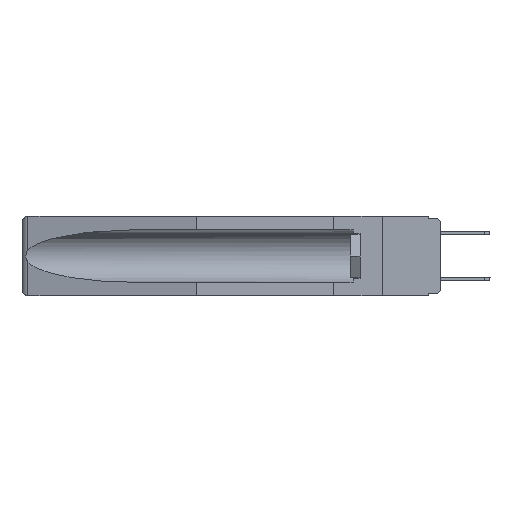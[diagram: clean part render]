
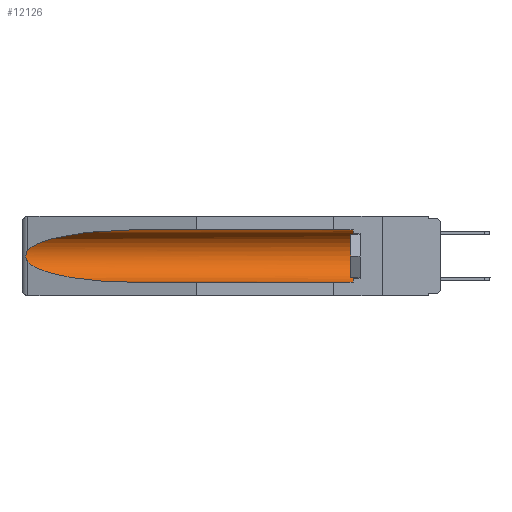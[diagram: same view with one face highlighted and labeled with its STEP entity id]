
A CAD part, left-side view. The second image highlights one B-rep face of the part: STEP entity #12126.
In plain terms, the highlighted cylindrical face has radius 2.857 mm (diameter 5.715 mm), a partial arc.
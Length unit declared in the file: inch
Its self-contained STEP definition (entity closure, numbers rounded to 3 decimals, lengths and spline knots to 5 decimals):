
#92 = CARTESIAN_POINT ( 'NONE',  ( 0.26597, 1.5296, -0.19026 ) ) ;
#160 = CARTESIAN_POINT ( 'NONE',  ( 0.2675, 1.53308, -0.17534 ) ) ;
#314 = CARTESIAN_POINT ( 'NONE',  ( 0.21114, 1.30732, -0.284 ) ) ;
#793 = CARTESIAN_POINT ( 'NONE',  ( 0.26537, 1.52718, -0.14972 ) ) ;
#815 = VERTEX_POINT ( 'NONE', #5006 ) ;
#1790 = CARTESIAN_POINT ( 'NONE',  ( 0.2673, 1.5327, -0.16383 ) ) ;
#1951 = CARTESIAN_POINT ( 'NONE',  ( 0.155, 1.07973, -0.284 ) ) ;
#2643 = CIRCLE ( 'NONE', #19537, 0.1125 ) ;
#2951 = CARTESIAN_POINT ( 'NONE',  ( 0.155, 0.126, -0.1715 ) ) ;
#3215 = CARTESIAN_POINT ( 'NONE',  ( 0.155, -0.30754, -0.1715 ) ) ;
#3278 = LINE ( 'NONE', #11334, #18023 ) ;
#3651 = VERTEX_POINT ( 'NONE', #17450 ) ;
#4057 = VERTEX_POINT ( 'NONE', #12811 ) ;
#5006 = CARTESIAN_POINT ( 'NONE',  ( 0.155, 0.126, -0.059 ) ) ;
#6608 = DIRECTION ( 'NONE',  ( 0., 1., 0. ) ) ;
#6919 = CARTESIAN_POINT ( 'NONE',  ( 0.2675, 1.53308, -0.16763 ) ) ;
#7635 = ORIENTED_EDGE ( 'NONE', *, *, #14720, .T. ) ;
#7788 = ORIENTED_EDGE ( 'NONE', *, *, #12703, .T. ) ;
#8964 = VECTOR ( 'NONE', #14452, 39.37008 ) ;
#8968 =( BOUNDED_CURVE ( )  B_SPLINE_CURVE ( 3, ( #12508, #19167, #314, #1951 ),
 .UNSPECIFIED., .F., .F. ) 
 B_SPLINE_CURVE_WITH_KNOTS ( ( 4, 4 ),
 ( 0.1948, 1.5708 ),
 .UNSPECIFIED. ) 
 CURVE ( )  GEOMETRIC_REPRESENTATION_ITEM ( )  RATIONAL_B_SPLINE_CURVE ( ( 1., 0.848, 0.848, 1. ) ) 
 REPRESENTATION_ITEM ( '' )  );
#9382 = CARTESIAN_POINT ( 'NONE',  ( 0.21114, 1.30732, -0.059 ) ) ;
#10629 = CARTESIAN_POINT ( 'NONE',  ( 0.26537, 1.52718, -0.14972 ) ) ;
#10839 = VERTEX_POINT ( 'NONE', #17985 ) ;
#11134 = CARTESIAN_POINT ( 'NONE',  ( 0.25451, 1.48313, -0.09465 ) ) ;
#11334 = CARTESIAN_POINT ( 'NONE',  ( 0.155, -0.30754, -0.284 ) ) ;
#11445 = ORIENTED_EDGE ( 'NONE', *, *, #18980, .F. ) ;
#12054 = CARTESIAN_POINT ( 'NONE',  ( 0.26597, 1.52961, -0.15275 ) ) ;
#12126 = ADVANCED_FACE ( 'NONE', ( #15658 ), #19638, .F. ) ;
#12508 = CARTESIAN_POINT ( 'NONE',  ( 0.26537, 1.52718, -0.19328 ) ) ;
#12614 = CARTESIAN_POINT ( 'NONE',  ( 0.155, -0.30754, -0.059 ) ) ;
#12703 = EDGE_CURVE ( 'NONE', #815, #10839, #21797, .T. ) ;
#12811 = CARTESIAN_POINT ( 'NONE',  ( 0.26537, 1.52718, -0.19328 ) ) ;
#12832 = CARTESIAN_POINT ( 'NONE',  ( 0.155, 0.126, -0.284 ) ) ;
#12970 =( BOUNDED_CURVE ( )  B_SPLINE_CURVE ( 3, ( #19812, #9382, #11134, #793 ),
 .UNSPECIFIED., .F., .F. ) 
 B_SPLINE_CURVE_WITH_KNOTS ( ( 4, 4 ),
 ( 4.71239, 6.08839 ),
 .UNSPECIFIED. ) 
 CURVE ( )  GEOMETRIC_REPRESENTATION_ITEM ( )  RATIONAL_B_SPLINE_CURVE ( ( 1., 0.848, 0.848, 1. ) ) 
 REPRESENTATION_ITEM ( '' )  );
#13004 = ORIENTED_EDGE ( 'NONE', *, *, #19296, .T. ) ;
#13380 = DIRECTION ( 'NONE',  ( 0., 0., 1. ) ) ;
#13410 = DIRECTION ( 'NONE',  ( 0., -1., 0. ) ) ;
#13753 = CARTESIAN_POINT ( 'NONE',  ( 0.26654, 1.53092, -0.15636 ) ) ;
#13921 = B_SPLINE_CURVE_WITH_KNOTS ( 'NONE', 3,
 ( #10629, #12054, #13753, #1790, #6919, #160, #17448, #18860, #92, #15694 ),
 .UNSPECIFIED., .F., .F.,
 ( 4, 2, 2, 2, 4 ),
 ( 0., 0.00029, 0.00058, 0.00087, 0.00117 ),
 .UNSPECIFIED. ) ;
#14192 = ORIENTED_EDGE ( 'NONE', *, *, #16176, .T. ) ;
#14452 = DIRECTION ( 'NONE',  ( 0., 1., 0. ) ) ;
#14486 = CARTESIAN_POINT ( 'NONE',  ( 0.26537, 1.52718, -0.14972 ) ) ;
#14559 = VERTEX_POINT ( 'NONE', #12832 ) ;
#14720 = EDGE_CURVE ( 'NONE', #14559, #815, #2643, .T. ) ;
#15120 = DIRECTION ( 'NONE',  ( 0., 0., 1. ) ) ;
#15327 = EDGE_CURVE ( 'NONE', #17410, #4057, #13921, .T. ) ;
#15658 = FACE_OUTER_BOUND ( 'NONE', #20547, .T. ) ;
#15694 = CARTESIAN_POINT ( 'NONE',  ( 0.26537, 1.52718, -0.19328 ) ) ;
#16176 = EDGE_CURVE ( 'NONE', #10839, #17410, #12970, .T. ) ;
#16674 = DIRECTION ( 'NONE',  ( 0., 1., 0. ) ) ;
#17410 = VERTEX_POINT ( 'NONE', #14486 ) ;
#17448 = CARTESIAN_POINT ( 'NONE',  ( 0.2673, 1.53269, -0.17917 ) ) ;
#17450 = CARTESIAN_POINT ( 'NONE',  ( 0.155, 1.07973, -0.284 ) ) ;
#17985 = CARTESIAN_POINT ( 'NONE',  ( 0.155, 1.07973, -0.059 ) ) ;
#18023 = VECTOR ( 'NONE', #16674, 39.37008 ) ;
#18481 = AXIS2_PLACEMENT_3D ( 'NONE', #3215, #6608, #13380 ) ;
#18860 = CARTESIAN_POINT ( 'NONE',  ( 0.26655, 1.53094, -0.18657 ) ) ;
#18980 = EDGE_CURVE ( 'NONE', #14559, #3651, #3278, .T. ) ;
#19167 = CARTESIAN_POINT ( 'NONE',  ( 0.25451, 1.48313, -0.24835 ) ) ;
#19296 = EDGE_CURVE ( 'NONE', #4057, #3651, #8968, .T. ) ;
#19537 = AXIS2_PLACEMENT_3D ( 'NONE', #2951, #13410, #15120 ) ;
#19638 = CYLINDRICAL_SURFACE ( 'NONE', #18481, 0.1125 ) ;
#19812 = CARTESIAN_POINT ( 'NONE',  ( 0.155, 1.07973, -0.059 ) ) ;
#20547 = EDGE_LOOP ( 'NONE', ( #14192, #21752, #13004, #11445, #7635, #7788 ) ) ;
#21752 = ORIENTED_EDGE ( 'NONE', *, *, #15327, .T. ) ;
#21797 = LINE ( 'NONE', #12614, #8964 ) ;
